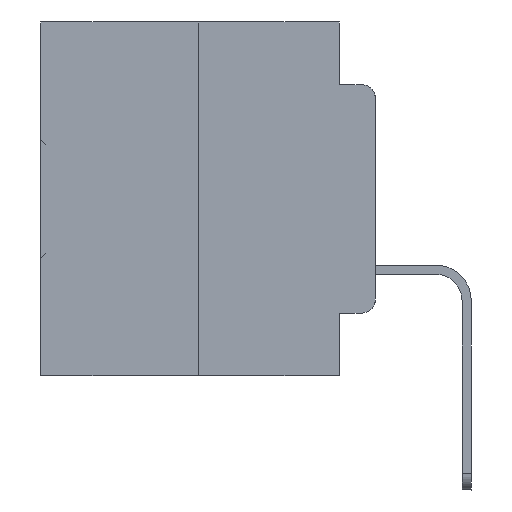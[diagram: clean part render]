
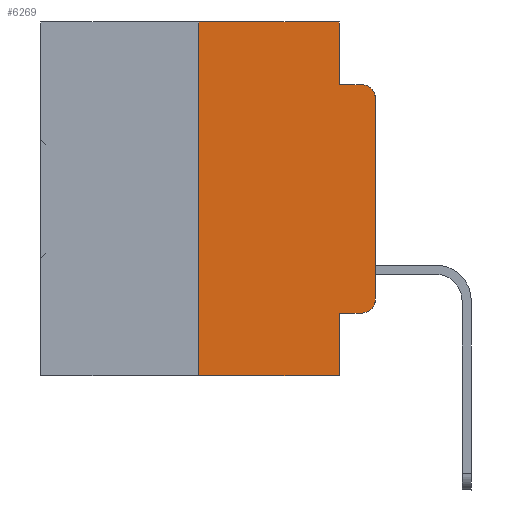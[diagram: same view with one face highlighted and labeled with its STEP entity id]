
A CAD part, left-side view. The second image highlights one B-rep face of the part: STEP entity #6269.
In plain terms, the highlighted planar face has unit normal (-1, 0, 0).
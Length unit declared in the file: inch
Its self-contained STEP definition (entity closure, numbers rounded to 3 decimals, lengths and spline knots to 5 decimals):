
#182 = EDGE_CURVE ( 'NONE', #17417, #18048, #9655, .T. ) ;
#919 = FACE_OUTER_BOUND ( 'NONE', #20650, .T. ) ;
#1024 = VECTOR ( 'NONE', #26237, 39.37008 ) ;
#1250 = CIRCLE ( 'NONE', #6430, 0.02 ) ;
#1452 = DIRECTION ( 'NONE',  ( 0., 0., -1. ) ) ;
#1752 = DIRECTION ( 'NONE',  ( 1., 0., 0. ) ) ;
#2170 = EDGE_CURVE ( 'NONE', #25813, #3117, #9596, .T. ) ;
#2270 = ORIENTED_EDGE ( 'NONE', *, *, #2170, .T. ) ;
#2809 = VECTOR ( 'NONE', #28782, 39.37008 ) ;
#3117 = VERTEX_POINT ( 'NONE', #28128 ) ;
#3395 = CARTESIAN_POINT ( 'NONE',  ( 0., 0.473, 0. ) ) ;
#4190 = ORIENTED_EDGE ( 'NONE', *, *, #11201, .F. ) ;
#5029 = DIRECTION ( 'NONE',  ( 0., 0., 1. ) ) ;
#6269 = ADVANCED_FACE ( 'NONE', ( #919 ), #19322, .F. ) ;
#6377 = LINE ( 'NONE', #29180, #7649 ) ;
#6430 = AXIS2_PLACEMENT_3D ( 'NONE', #26272, #16239, #31579 ) ;
#6622 = CARTESIAN_POINT ( 'NONE',  ( 0., 0.02, -0.1085 ) ) ;
#6766 = DIRECTION ( 'NONE',  ( 0., 0., -1. ) ) ;
#6787 = ORIENTED_EDGE ( 'NONE', *, *, #182, .T. ) ;
#6984 = VECTOR ( 'NONE', #1452, 39.37008 ) ;
#7562 = VERTEX_POINT ( 'NONE', #23039 ) ;
#7563 = VECTOR ( 'NONE', #31804, 39.37008 ) ;
#7649 = VECTOR ( 'NONE', #23991, 39.37008 ) ;
#7784 = EDGE_CURVE ( 'NONE', #18166, #25813, #19939, .T. ) ;
#8651 = ORIENTED_EDGE ( 'NONE', *, *, #34153, .F. ) ;
#9596 = CIRCLE ( 'NONE', #17964, 0.02 ) ;
#9655 = LINE ( 'NONE', #18287, #7563 ) ;
#10062 = AXIS2_PLACEMENT_3D ( 'NONE', #3395, #1752, #6766 ) ;
#10822 = DIRECTION ( 'NONE',  ( 0., -1., 0. ) ) ;
#10847 = VECTOR ( 'NONE', #5029, 39.37008 ) ;
#11201 = EDGE_CURVE ( 'NONE', #31280, #15331, #6377, .T. ) ;
#11726 = EDGE_CURVE ( 'NONE', #32903, #31280, #23380, .T. ) ;
#11889 = LINE ( 'NONE', #28980, #1024 ) ;
#12758 = VERTEX_POINT ( 'NONE', #27447 ) ;
#13078 = EDGE_CURVE ( 'NONE', #12758, #18166, #1250, .T. ) ;
#14957 = CARTESIAN_POINT ( 'NONE',  ( 0., 0.473, 0. ) ) ;
#15151 = ORIENTED_EDGE ( 'NONE', *, *, #20425, .F. ) ;
#15331 = VERTEX_POINT ( 'NONE', #15579 ) ;
#15482 = LINE ( 'NONE', #18812, #22472 ) ;
#15579 = CARTESIAN_POINT ( 'NONE',  ( 0., 0.051, -0.0885 ) ) ;
#15726 = ORIENTED_EDGE ( 'NONE', *, *, #11726, .F. ) ;
#16171 = LINE ( 'NONE', #18192, #2809 ) ;
#16239 = DIRECTION ( 'NONE',  ( -1., 0., 0. ) ) ;
#17207 = VECTOR ( 'NONE', #28310, 39.37008 ) ;
#17417 = VERTEX_POINT ( 'NONE', #23657 ) ;
#17964 = AXIS2_PLACEMENT_3D ( 'NONE', #6622, #33262, #19878 ) ;
#18048 = VERTEX_POINT ( 'NONE', #23468 ) ;
#18166 = VERTEX_POINT ( 'NONE', #21382 ) ;
#18192 = CARTESIAN_POINT ( 'NONE',  ( 0., 0.25, 0. ) ) ;
#18287 = CARTESIAN_POINT ( 'NONE',  ( 0., 0.473, -0.5 ) ) ;
#18304 = CARTESIAN_POINT ( 'NONE',  ( 0., 0., 0. ) ) ;
#18443 = ORIENTED_EDGE ( 'NONE', *, *, #33736, .T. ) ;
#18812 = CARTESIAN_POINT ( 'NONE',  ( 0., 0.051, -0.0885 ) ) ;
#19322 = PLANE ( 'NONE',  #10062 ) ;
#19878 = DIRECTION ( 'NONE',  ( 0., 0., -1. ) ) ;
#19928 = CARTESIAN_POINT ( 'NONE',  ( 0., 0.25, 0. ) ) ;
#19939 = LINE ( 'NONE', #18304, #10847 ) ;
#20425 = EDGE_CURVE ( 'NONE', #15331, #3117, #15482, .T. ) ;
#20650 = EDGE_LOOP ( 'NONE', ( #21524, #2270, #15151, #4190, #15726, #8651, #6787, #34120, #18443, #24021 ) ) ;
#21382 = CARTESIAN_POINT ( 'NONE',  ( 0., 0., -0.3915 ) ) ;
#21524 = ORIENTED_EDGE ( 'NONE', *, *, #7784, .T. ) ;
#21547 = LINE ( 'NONE', #33316, #6984 ) ;
#22472 = VECTOR ( 'NONE', #10822, 39.37008 ) ;
#23039 = CARTESIAN_POINT ( 'NONE',  ( 0., 0.051, -0.4115 ) ) ;
#23380 = LINE ( 'NONE', #14957, #17207 ) ;
#23468 = CARTESIAN_POINT ( 'NONE',  ( 0., 0.051, -0.5 ) ) ;
#23657 = CARTESIAN_POINT ( 'NONE',  ( 0., 0.25, -0.5 ) ) ;
#23991 = DIRECTION ( 'NONE',  ( 0., 0., -1. ) ) ;
#24021 = ORIENTED_EDGE ( 'NONE', *, *, #13078, .T. ) ;
#25813 = VERTEX_POINT ( 'NONE', #32468 ) ;
#26237 = DIRECTION ( 'NONE',  ( 0., -1., 0. ) ) ;
#26272 = CARTESIAN_POINT ( 'NONE',  ( 0., 0.02, -0.3915 ) ) ;
#27447 = CARTESIAN_POINT ( 'NONE',  ( 0., 0.02, -0.4115 ) ) ;
#28128 = CARTESIAN_POINT ( 'NONE',  ( 0., 0.02, -0.0885 ) ) ;
#28310 = DIRECTION ( 'NONE',  ( 0., -1., 0. ) ) ;
#28782 = DIRECTION ( 'NONE',  ( 0., 0., 1. ) ) ;
#28980 = CARTESIAN_POINT ( 'NONE',  ( 0., 0.051, -0.4115 ) ) ;
#29180 = CARTESIAN_POINT ( 'NONE',  ( 0., 0.051, 0. ) ) ;
#29468 = CARTESIAN_POINT ( 'NONE',  ( 0., 0.051, 0. ) ) ;
#31280 = VERTEX_POINT ( 'NONE', #29468 ) ;
#31579 = DIRECTION ( 'NONE',  ( 0., 0., -1. ) ) ;
#31804 = DIRECTION ( 'NONE',  ( 0., -1., 0. ) ) ;
#32468 = CARTESIAN_POINT ( 'NONE',  ( 0., 0., -0.1085 ) ) ;
#32903 = VERTEX_POINT ( 'NONE', #19928 ) ;
#33262 = DIRECTION ( 'NONE',  ( -1., 0., 0. ) ) ;
#33316 = CARTESIAN_POINT ( 'NONE',  ( 0., 0.051, 0. ) ) ;
#33736 = EDGE_CURVE ( 'NONE', #7562, #12758, #11889, .T. ) ;
#33989 = EDGE_CURVE ( 'NONE', #7562, #18048, #21547, .T. ) ;
#34120 = ORIENTED_EDGE ( 'NONE', *, *, #33989, .F. ) ;
#34153 = EDGE_CURVE ( 'NONE', #17417, #32903, #16171, .T. ) ;
